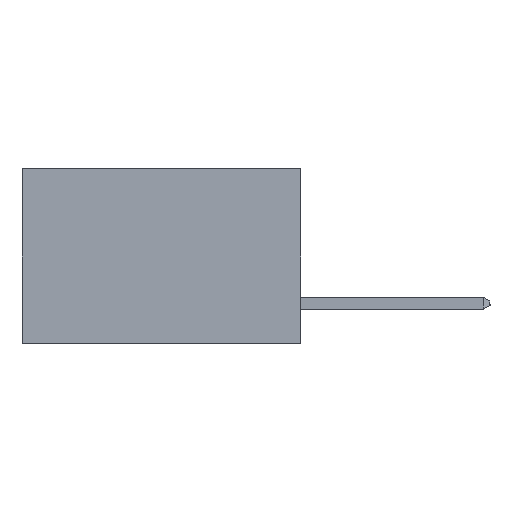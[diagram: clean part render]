
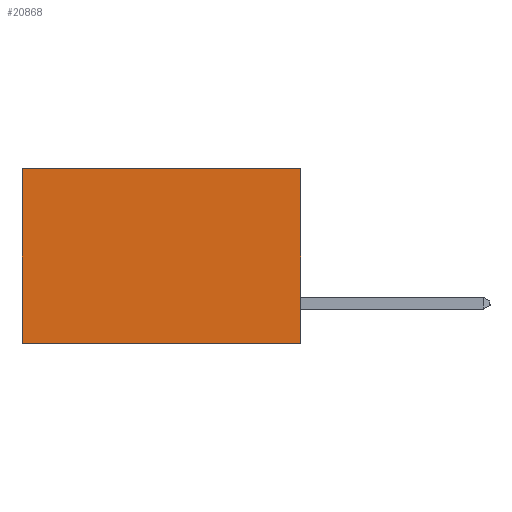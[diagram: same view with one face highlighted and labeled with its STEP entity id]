
A CAD part, left-side view. The second image highlights one B-rep face of the part: STEP entity #20868.
In plain terms, the highlighted planar face has unit normal (-1, 0, 0).
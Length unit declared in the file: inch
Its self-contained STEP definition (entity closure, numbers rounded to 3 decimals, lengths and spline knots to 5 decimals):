
#282 = CARTESIAN_POINT ( 'NONE',  ( 0.277, 0., 0. ) ) ;
#1790 = EDGE_LOOP ( 'NONE', ( #5473, #14505, #15672, #12628 ) ) ;
#1990 = EDGE_CURVE ( 'NONE', #2215, #14913, #9989, .T. ) ;
#2215 = VERTEX_POINT ( 'NONE', #3125 ) ;
#2810 = VERTEX_POINT ( 'NONE', #18840 ) ;
#2978 = DIRECTION ( 'NONE',  ( 1., 0., 0. ) ) ;
#3125 = CARTESIAN_POINT ( 'NONE',  ( 0.277, 0.59, 0. ) ) ;
#3974 = CARTESIAN_POINT ( 'NONE',  ( 0.277, 0.59, -0.37 ) ) ;
#4717 = CARTESIAN_POINT ( 'NONE',  ( 0.277, 0., -0.37 ) ) ;
#5448 = VECTOR ( 'NONE', #17049, 39.37008 ) ;
#5473 = ORIENTED_EDGE ( 'NONE', *, *, #1990, .T. ) ;
#5648 = CARTESIAN_POINT ( 'NONE',  ( 0.277, 0., -0.37 ) ) ;
#6974 = CARTESIAN_POINT ( 'NONE',  ( 0.277, 0., 0. ) ) ;
#7360 = DIRECTION ( 'NONE',  ( 0., 1., 0. ) ) ;
#7495 = AXIS2_PLACEMENT_3D ( 'NONE', #4717, #2978, #14833 ) ;
#9495 = CARTESIAN_POINT ( 'NONE',  ( 0.277, 0.59, -0.37 ) ) ;
#9578 = LINE ( 'NONE', #6974, #19377 ) ;
#9989 = LINE ( 'NONE', #9495, #5448 ) ;
#10468 = VECTOR ( 'NONE', #11658, 39.37008 ) ;
#10545 = EDGE_CURVE ( 'NONE', #16837, #2810, #14854, .T. ) ;
#11658 = DIRECTION ( 'NONE',  ( 0., 0., -1. ) ) ;
#12422 = EDGE_CURVE ( 'NONE', #2810, #14913, #15511, .T. ) ;
#12628 = ORIENTED_EDGE ( 'NONE', *, *, #12923, .T. ) ;
#12923 = EDGE_CURVE ( 'NONE', #16837, #2215, #9578, .T. ) ;
#13180 = PLANE ( 'NONE',  #7495 ) ;
#14505 = ORIENTED_EDGE ( 'NONE', *, *, #12422, .F. ) ;
#14833 = DIRECTION ( 'NONE',  ( 0., 0., -1. ) ) ;
#14854 = LINE ( 'NONE', #18194, #10468 ) ;
#14913 = VERTEX_POINT ( 'NONE', #3974 ) ;
#15511 = LINE ( 'NONE', #5648, #19919 ) ;
#15672 = ORIENTED_EDGE ( 'NONE', *, *, #10545, .F. ) ;
#16837 = VERTEX_POINT ( 'NONE', #282 ) ;
#17049 = DIRECTION ( 'NONE',  ( 0., 0., -1. ) ) ;
#18194 = CARTESIAN_POINT ( 'NONE',  ( 0.277, 0., -0.37 ) ) ;
#18572 = DIRECTION ( 'NONE',  ( 0., 1., 0. ) ) ;
#18840 = CARTESIAN_POINT ( 'NONE',  ( 0.277, 0., -0.37 ) ) ;
#19377 = VECTOR ( 'NONE', #18572, 39.37008 ) ;
#19919 = VECTOR ( 'NONE', #7360, 39.37008 ) ;
#20054 = FACE_OUTER_BOUND ( 'NONE', #1790, .T. ) ;
#20868 = ADVANCED_FACE ( 'NONE', ( #20054 ), #13180, .F. ) ;
